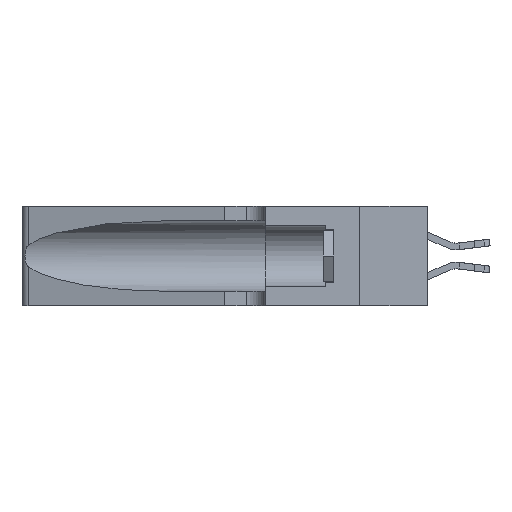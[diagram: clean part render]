
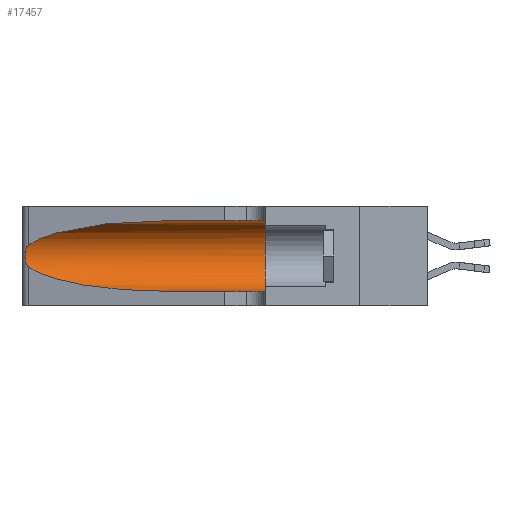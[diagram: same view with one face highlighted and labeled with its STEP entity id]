
A CAD part, left-side view. The second image highlights one B-rep face of the part: STEP entity #17457.
In plain terms, the highlighted cylindrical face has radius 3.308 mm (diameter 6.617 mm), a partial arc.
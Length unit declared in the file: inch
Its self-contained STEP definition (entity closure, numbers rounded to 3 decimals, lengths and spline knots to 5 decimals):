
#223 = VECTOR ( 'NONE', #6241, 39.37008 ) ;
#299 = CARTESIAN_POINT ( 'NONE',  ( 0.1305, 0.72297, 0.05475 ) ) ;
#396 =( BOUNDED_CURVE ( )  B_SPLINE_CURVE ( 3, ( #17850, #1109, #3222, #19938 ),
 .UNSPECIFIED., .F., .F. ) 
 B_SPLINE_CURVE_WITH_KNOTS ( ( 4, 4 ),
 ( 1.5708, 2.84003 ),
 .UNSPECIFIED. ) 
 CURVE ( )  GEOMETRIC_REPRESENTATION_ITEM ( )  RATIONAL_B_SPLINE_CURVE ( ( 1., 0.87, 0.87, 1. ) ) 
 REPRESENTATION_ITEM ( '' )  );
#1003 = CARTESIAN_POINT ( 'NONE',  ( 0.25487, 1.22718, 0.14631 ) ) ;
#1109 = CARTESIAN_POINT ( 'NONE',  ( 0.18966, 0.96281, 0.31525 ) ) ;
#1182 = CARTESIAN_POINT ( 'NONE',  ( 0.1305, 0.35, 0.31525 ) ) ;
#2417 = VERTEX_POINT ( 'NONE', #9823 ) ;
#2816 = DIRECTION ( 'NONE',  ( 0., 1., 0. ) ) ;
#3019 = CARTESIAN_POINT ( 'NONE',  ( 0.25639, 1.23184, 0.21858 ) ) ;
#3222 = CARTESIAN_POINT ( 'NONE',  ( 0.2373, 1.15595, 0.28018 ) ) ;
#3712 = CARTESIAN_POINT ( 'NONE',  ( 0.1305, 0.72297, 0.31525 ) ) ;
#3959 = AXIS2_PLACEMENT_3D ( 'NONE', #15379, #2816, #17454 ) ;
#4023 = ORIENTED_EDGE ( 'NONE', *, *, #17388, .T. ) ;
#5146 = CARTESIAN_POINT ( 'NONE',  ( 0.25854, 1.2359, 0.20912 ) ) ;
#5796 = LINE ( 'NONE', #12496, #223 ) ;
#6241 = DIRECTION ( 'NONE',  ( 0., -1., 0. ) ) ;
#6359 = VERTEX_POINT ( 'NONE', #1182 ) ;
#6742 = LINE ( 'NONE', #22565, #23412 ) ;
#6754 = B_SPLINE_CURVE_WITH_KNOTS ( 'NONE', 3,
 ( #13482, #25937, #3019, #17649, #5146, #19746, #7247, #21826, #9366, #23956, #11474, #26017, #13568, #1003 ),
 .UNSPECIFIED., .F., .F.,
 ( 4, 2, 2, 2, 2, 2, 4 ),
 ( 0., 0.00027, 0.00053, 0.00107, 0.0016, 0.00187, 0.00214 ),
 .UNSPECIFIED. ) ;
#7247 = CARTESIAN_POINT ( 'NONE',  ( 0.26075, 1.23896, 0.19203 ) ) ;
#7574 = ORIENTED_EDGE ( 'NONE', *, *, #18237, .T. ) ;
#7676 = EDGE_CURVE ( 'NONE', #9083, #25939, #396, .T. ) ;
#7954 = DIRECTION ( 'NONE',  ( 0., -1., 0. ) ) ;
#8129 = ORIENTED_EDGE ( 'NONE', *, *, #23548, .F. ) ;
#8558 = CARTESIAN_POINT ( 'NONE',  ( 0.2373, 1.15595, 0.08982 ) ) ;
#8627 = ORIENTED_EDGE ( 'NONE', *, *, #7676, .T. ) ;
#9083 = VERTEX_POINT ( 'NONE', #3712 ) ;
#9366 = CARTESIAN_POINT ( 'NONE',  ( 0.26017, 1.23833, 0.17102 ) ) ;
#9823 = CARTESIAN_POINT ( 'NONE',  ( 0.1305, 0.72297, 0.05475 ) ) ;
#10875 = CARTESIAN_POINT ( 'NONE',  ( 0.25487, 1.22718, 0.22369 ) ) ;
#11474 = CARTESIAN_POINT ( 'NONE',  ( 0.25789, 1.23486, 0.15765 ) ) ;
#12182 = CARTESIAN_POINT ( 'NONE',  ( 0.1305, 1.61858, 0.185 ) ) ;
#12496 = CARTESIAN_POINT ( 'NONE',  ( 0.1305, 1.61858, 0.31525 ) ) ;
#12865 = CARTESIAN_POINT ( 'NONE',  ( 0.18966, 0.96281, 0.05475 ) ) ;
#13482 = CARTESIAN_POINT ( 'NONE',  ( 0.25487, 1.22718, 0.22369 ) ) ;
#13568 = CARTESIAN_POINT ( 'NONE',  ( 0.25555, 1.22993, 0.14849 ) ) ;
#13634 = CARTESIAN_POINT ( 'NONE',  ( 0.1305, 0.35, 0.05475 ) ) ;
#15379 = CARTESIAN_POINT ( 'NONE',  ( 0.1305, 0.35, 0.185 ) ) ;
#16133 = CARTESIAN_POINT ( 'NONE',  ( 0.25487, 1.22718, 0.14631 ) ) ;
#16432 = DIRECTION ( 'NONE',  ( 0., 0., -1. ) ) ;
#16462 =( BOUNDED_CURVE ( )  B_SPLINE_CURVE ( 3, ( #21117, #8558, #12865, #299 ),
 .UNSPECIFIED., .F., .F. ) 
 B_SPLINE_CURVE_WITH_KNOTS ( ( 4, 4 ),
 ( 3.44316, 4.71239 ),
 .UNSPECIFIED. ) 
 CURVE ( )  GEOMETRIC_REPRESENTATION_ITEM ( )  RATIONAL_B_SPLINE_CURVE ( ( 1., 0.87, 0.87, 1. ) ) 
 REPRESENTATION_ITEM ( '' )  );
#17388 = EDGE_CURVE ( 'NONE', #2417, #25494, #6742, .T. ) ;
#17454 = DIRECTION ( 'NONE',  ( 0., 0., 1. ) ) ;
#17457 = ADVANCED_FACE ( 'NONE', ( #21415 ), #20759, .F. ) ;
#17649 = CARTESIAN_POINT ( 'NONE',  ( 0.25787, 1.23484, 0.2124 ) ) ;
#17850 = CARTESIAN_POINT ( 'NONE',  ( 0.1305, 0.72297, 0.31525 ) ) ;
#18091 = ORIENTED_EDGE ( 'NONE', *, *, #21885, .T. ) ;
#18237 = EDGE_CURVE ( 'NONE', #26301, #2417, #16462, .T. ) ;
#18406 = EDGE_LOOP ( 'NONE', ( #8627, #18091, #7574, #4023, #21351, #8129 ) ) ;
#19746 = CARTESIAN_POINT ( 'NONE',  ( 0.26018, 1.23835, 0.19895 ) ) ;
#19749 = EDGE_CURVE ( 'NONE', #6359, #25494, #20001, .T. ) ;
#19938 = CARTESIAN_POINT ( 'NONE',  ( 0.25487, 1.22718, 0.22369 ) ) ;
#20001 = CIRCLE ( 'NONE', #3959, 0.13025 ) ;
#20759 = CYLINDRICAL_SURFACE ( 'NONE', #24906, 0.13025 ) ;
#21117 = CARTESIAN_POINT ( 'NONE',  ( 0.25487, 1.22718, 0.14631 ) ) ;
#21351 = ORIENTED_EDGE ( 'NONE', *, *, #19749, .F. ) ;
#21415 = FACE_OUTER_BOUND ( 'NONE', #18406, .T. ) ;
#21826 = CARTESIAN_POINT ( 'NONE',  ( 0.26075, 1.23896, 0.178 ) ) ;
#21885 = EDGE_CURVE ( 'NONE', #25939, #26301, #6754, .T. ) ;
#22565 = CARTESIAN_POINT ( 'NONE',  ( 0.1305, 1.61858, 0.05475 ) ) ;
#23412 = VECTOR ( 'NONE', #7954, 39.37008 ) ;
#23548 = EDGE_CURVE ( 'NONE', #9083, #6359, #5796, .T. ) ;
#23956 = CARTESIAN_POINT ( 'NONE',  ( 0.25856, 1.23593, 0.16098 ) ) ;
#24906 = AXIS2_PLACEMENT_3D ( 'NONE', #12182, #26867, #16432 ) ;
#25494 = VERTEX_POINT ( 'NONE', #13634 ) ;
#25937 = CARTESIAN_POINT ( 'NONE',  ( 0.25555, 1.22994, 0.2215 ) ) ;
#25939 = VERTEX_POINT ( 'NONE', #10875 ) ;
#26017 = CARTESIAN_POINT ( 'NONE',  ( 0.25639, 1.23186, 0.15144 ) ) ;
#26301 = VERTEX_POINT ( 'NONE', #16133 ) ;
#26867 = DIRECTION ( 'NONE',  ( 0., -1., 0. ) ) ;
